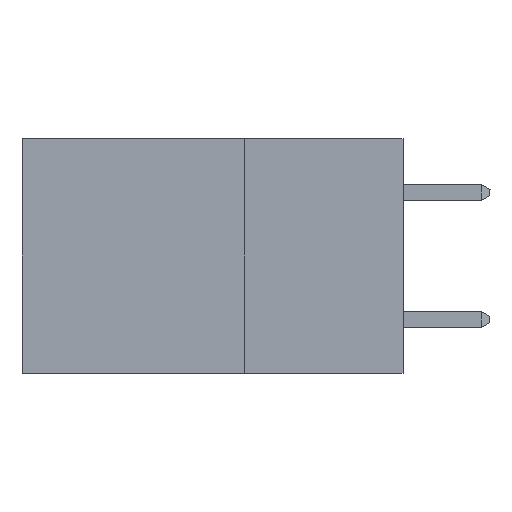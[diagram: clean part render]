
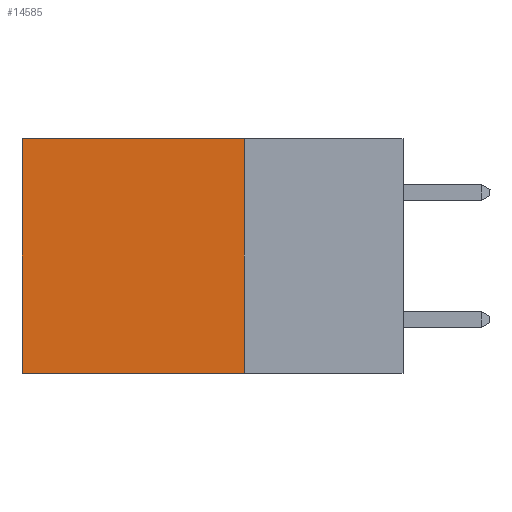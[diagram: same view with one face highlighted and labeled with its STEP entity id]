
A CAD part, left-side view. The second image highlights one B-rep face of the part: STEP entity #14585.
In plain terms, the highlighted planar face has unit normal (-1, 0, 0).
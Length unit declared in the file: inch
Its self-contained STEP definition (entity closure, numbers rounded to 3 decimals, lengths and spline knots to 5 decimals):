
#730 = CARTESIAN_POINT ( 'NONE',  ( 0.2875, 0.25, 0. ) ) ;
#2300 = PLANE ( 'NONE',  #3634 ) ;
#2355 = VERTEX_POINT ( 'NONE', #38205 ) ;
#3634 = AXIS2_PLACEMENT_3D ( 'NONE', #9216, #33691, #12807 ) ;
#4172 = DIRECTION ( 'NONE',  ( 0., 1., 0. ) ) ;
#4662 = CARTESIAN_POINT ( 'NONE',  ( 0.2875, 0.25, 0. ) ) ;
#8513 = FACE_OUTER_BOUND ( 'NONE', #28764, .T. ) ;
#9216 = CARTESIAN_POINT ( 'NONE',  ( 0.2875, 0.25, 0. ) ) ;
#9928 = LINE ( 'NONE', #4662, #28509 ) ;
#10566 = DIRECTION ( 'NONE',  ( 0., 0., -1. ) ) ;
#11658 = EDGE_CURVE ( 'NONE', #22151, #26541, #9928, .T. ) ;
#12496 = LINE ( 'NONE', #31454, #40393 ) ;
#12807 = DIRECTION ( 'NONE',  ( 0., 0., -1. ) ) ;
#14585 = ADVANCED_FACE ( 'NONE', ( #8513 ), #2300, .F. ) ;
#16265 = VERTEX_POINT ( 'NONE', #32527 ) ;
#16936 = ORIENTED_EDGE ( 'NONE', *, *, #28486, .T. ) ;
#17567 = CARTESIAN_POINT ( 'NONE',  ( 0.2875, 0.25, -0.37 ) ) ;
#18586 = ORIENTED_EDGE ( 'NONE', *, *, #11658, .F. ) ;
#19612 = VECTOR ( 'NONE', #4172, 39.37008 ) ;
#20740 = LINE ( 'NONE', #730, #19612 ) ;
#21730 = LINE ( 'NONE', #17567, #29727 ) ;
#21879 = CARTESIAN_POINT ( 'NONE',  ( 0.2875, 0.25, 0. ) ) ;
#22151 = VERTEX_POINT ( 'NONE', #21879 ) ;
#24582 = ORIENTED_EDGE ( 'NONE', *, *, #35652, .F. ) ;
#25077 = ORIENTED_EDGE ( 'NONE', *, *, #33708, .T. ) ;
#26541 = VERTEX_POINT ( 'NONE', #32830 ) ;
#27932 = DIRECTION ( 'NONE',  ( 0., 1., 0. ) ) ;
#28486 = EDGE_CURVE ( 'NONE', #22151, #2355, #20740, .T. ) ;
#28509 = VECTOR ( 'NONE', #29042, 39.37008 ) ;
#28764 = EDGE_LOOP ( 'NONE', ( #25077, #24582, #18586, #16936 ) ) ;
#29042 = DIRECTION ( 'NONE',  ( 0., 0., -1. ) ) ;
#29727 = VECTOR ( 'NONE', #27932, 39.37008 ) ;
#31454 = CARTESIAN_POINT ( 'NONE',  ( 0.2875, 0.6, 0. ) ) ;
#32527 = CARTESIAN_POINT ( 'NONE',  ( 0.2875, 0.6, -0.37 ) ) ;
#32830 = CARTESIAN_POINT ( 'NONE',  ( 0.2875, 0.25, -0.37 ) ) ;
#33691 = DIRECTION ( 'NONE',  ( 1., 0., 0. ) ) ;
#33708 = EDGE_CURVE ( 'NONE', #2355, #16265, #12496, .T. ) ;
#35652 = EDGE_CURVE ( 'NONE', #26541, #16265, #21730, .T. ) ;
#38205 = CARTESIAN_POINT ( 'NONE',  ( 0.2875, 0.6, 0. ) ) ;
#40393 = VECTOR ( 'NONE', #10566, 39.37008 ) ;
